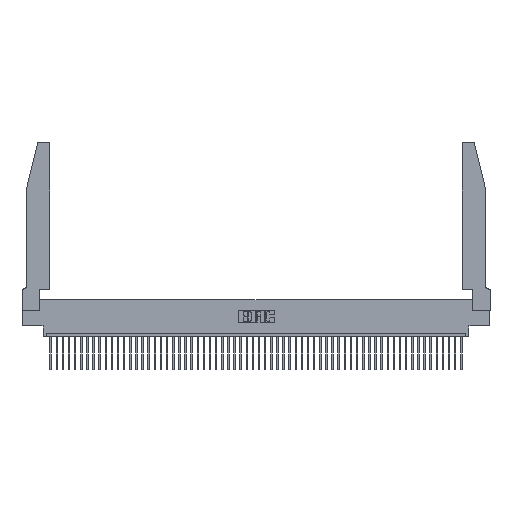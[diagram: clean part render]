
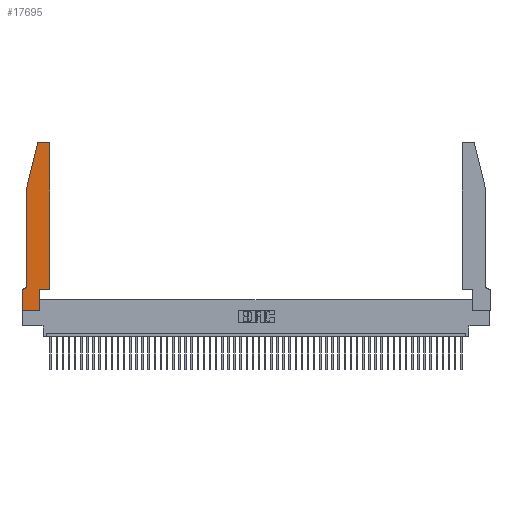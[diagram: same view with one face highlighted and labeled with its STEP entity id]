
A CAD part, top view. The second image highlights one B-rep face of the part: STEP entity #17695.
In plain terms, the highlighted planar face has unit normal (0, 0, 1).
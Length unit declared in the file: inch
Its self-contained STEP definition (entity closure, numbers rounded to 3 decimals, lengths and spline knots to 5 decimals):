
#689 = ORIENTED_EDGE ( 'NONE', *, *, #12841, .T. ) ;
#898 = DIRECTION ( 'NONE',  ( 0., 0., 1. ) ) ;
#978 = CARTESIAN_POINT ( 'NONE',  ( 0., 0., 0.37 ) ) ;
#1349 = CARTESIAN_POINT ( 'NONE',  ( 0.0755, 2., 0.37 ) ) ;
#2173 = CARTESIAN_POINT ( 'NONE',  ( 0.0755, 0.42, 0.37 ) ) ;
#2693 = DIRECTION ( 'NONE',  ( 0., 0., 1. ) ) ;
#2873 = VECTOR ( 'NONE', #14206, 39.37008 ) ;
#4176 = CIRCLE ( 'NONE', #28029, 0.03 ) ;
#4254 = CARTESIAN_POINT ( 'NONE',  ( 0., 0., 0.37 ) ) ;
#4898 = LINE ( 'NONE', #13164, #34151 ) ;
#6686 = VERTEX_POINT ( 'NONE', #15006 ) ;
#6772 = DIRECTION ( 'NONE',  ( 1., 0., 0. ) ) ;
#8226 = ORIENTED_EDGE ( 'NONE', *, *, #20039, .T. ) ;
#8615 = ORIENTED_EDGE ( 'NONE', *, *, #48968, .T. ) ;
#8838 = CARTESIAN_POINT ( 'NONE',  ( 0.2865, 0.35, 0.37 ) ) ;
#10948 = ORIENTED_EDGE ( 'NONE', *, *, #19358, .T. ) ;
#11020 = DIRECTION ( 'NONE',  ( 1., 0., 0. ) ) ;
#11480 = VECTOR ( 'NONE', #26104, 39.37008 ) ;
#11976 = EDGE_CURVE ( 'NONE', #18984, #33831, #35583, .T. ) ;
#12631 = FACE_OUTER_BOUND ( 'NONE', #30611, .T. ) ;
#12687 = CARTESIAN_POINT ( 'NONE',  ( 0.2605, 2.75, 0.37 ) ) ;
#12841 = EDGE_CURVE ( 'NONE', #29000, #18984, #4898, .T. ) ;
#13164 = CARTESIAN_POINT ( 'NONE',  ( 0.2865, 0.35, 0.37 ) ) ;
#13382 = VECTOR ( 'NONE', #45969, 39.37008 ) ;
#13775 = ORIENTED_EDGE ( 'NONE', *, *, #36613, .T. ) ;
#14206 = DIRECTION ( 'NONE',  ( 1., 0., 0. ) ) ;
#14802 = DIRECTION ( 'NONE',  ( 1., 0., 0. ) ) ;
#15006 = CARTESIAN_POINT ( 'NONE',  ( 0.0055, 0.35, 0.37 ) ) ;
#15253 = CARTESIAN_POINT ( 'NONE',  ( 0.4205, 2.72, 0.37 ) ) ;
#15315 = CARTESIAN_POINT ( 'NONE',  ( 0., 0.35, 0.37 ) ) ;
#16146 = DIRECTION ( 'NONE',  ( 0., 0., -1. ) ) ;
#16228 = VERTEX_POINT ( 'NONE', #49581 ) ;
#16940 = AXIS2_PLACEMENT_3D ( 'NONE', #43182, #2693, #6772 ) ;
#17523 = LINE ( 'NONE', #24568, #25081 ) ;
#17695 = ADVANCED_FACE ( 'NONE', ( #12631 ), #18202, .T. ) ;
#17924 = CARTESIAN_POINT ( 'NONE',  ( 0.0755, 2., 0.37 ) ) ;
#18202 = PLANE ( 'NONE',  #19454 ) ;
#18301 = EDGE_CURVE ( 'NONE', #24380, #6686, #25155, .T. ) ;
#18719 = VECTOR ( 'NONE', #29049, 39.37008 ) ;
#18984 = VERTEX_POINT ( 'NONE', #8838 ) ;
#19358 = EDGE_CURVE ( 'NONE', #36902, #28994, #4176, .T. ) ;
#19454 = AXIS2_PLACEMENT_3D ( 'NONE', #52340, #898, #14802 ) ;
#19615 = ORIENTED_EDGE ( 'NONE', *, *, #11976, .T. ) ;
#20039 = EDGE_CURVE ( 'NONE', #51931, #29000, #47998, .T. ) ;
#20915 = EDGE_CURVE ( 'NONE', #23450, #16228, #42098, .T. ) ;
#22613 = CARTESIAN_POINT ( 'NONE',  ( 0.284, 2.75, 0.37 ) ) ;
#23111 = DIRECTION ( 'NONE',  ( 0., 0., 1. ) ) ;
#23450 = VERTEX_POINT ( 'NONE', #22613 ) ;
#24380 = VERTEX_POINT ( 'NONE', #2173 ) ;
#24568 = CARTESIAN_POINT ( 'NONE',  ( 0.0755, 0.35, 0.37 ) ) ;
#25081 = VECTOR ( 'NONE', #33972, 39.37008 ) ;
#25155 = CIRCLE ( 'NONE', #28321, 0.07 ) ;
#25313 = ORIENTED_EDGE ( 'NONE', *, *, #18301, .T. ) ;
#25904 = CARTESIAN_POINT ( 'NONE',  ( 0., 0., 0.37 ) ) ;
#25976 = DIRECTION ( 'NONE',  ( 0., 1., 0. ) ) ;
#26104 = DIRECTION ( 'NONE',  ( 0., 1., 0. ) ) ;
#26651 = LINE ( 'NONE', #17924, #49461 ) ;
#27323 = CARTESIAN_POINT ( 'NONE',  ( 0.4505, 0.35, 0.37 ) ) ;
#28029 = AXIS2_PLACEMENT_3D ( 'NONE', #15253, #23111, #11020 ) ;
#28321 = AXIS2_PLACEMENT_3D ( 'NONE', #42640, #16146, #32679 ) ;
#28559 = ORIENTED_EDGE ( 'NONE', *, *, #45787, .T. ) ;
#28994 = VERTEX_POINT ( 'NONE', #38900 ) ;
#29000 = VERTEX_POINT ( 'NONE', #51292 ) ;
#29049 = DIRECTION ( 'NONE',  ( -1., 0., 0. ) ) ;
#29093 = LINE ( 'NONE', #978, #31085 ) ;
#30507 = DIRECTION ( 'NONE',  ( 0., -1., 0. ) ) ;
#30611 = EDGE_LOOP ( 'NONE', ( #28559, #51574, #41294, #13775, #25313, #48264, #52127, #8226, #689, #19615, #8615, #10948 ) ) ;
#31085 = VECTOR ( 'NONE', #30507, 39.37008 ) ;
#32187 = EDGE_CURVE ( 'NONE', #45238, #51931, #29093, .T. ) ;
#32679 = DIRECTION ( 'NONE',  ( -1., 0., 0. ) ) ;
#33831 = VERTEX_POINT ( 'NONE', #50479 ) ;
#33949 = EDGE_CURVE ( 'NONE', #6686, #45238, #17523, .T. ) ;
#33972 = DIRECTION ( 'NONE',  ( -1., 0., 0. ) ) ;
#34151 = VECTOR ( 'NONE', #25976, 39.37008 ) ;
#35583 = LINE ( 'NONE', #27323, #41892 ) ;
#36613 = EDGE_CURVE ( 'NONE', #42756, #24380, #47185, .T. ) ;
#36902 = VERTEX_POINT ( 'NONE', #46282 ) ;
#38220 = CARTESIAN_POINT ( 'NONE',  ( 0.4505, 0.35, 0.37 ) ) ;
#38408 = DIRECTION ( 'NONE',  ( -0.239, -0.971, 0. ) ) ;
#38900 = CARTESIAN_POINT ( 'NONE',  ( 0.4205, 2.75, 0.37 ) ) ;
#41294 = ORIENTED_EDGE ( 'NONE', *, *, #48977, .T. ) ;
#41892 = VECTOR ( 'NONE', #43498, 39.37008 ) ;
#42098 = CIRCLE ( 'NONE', #16940, 0.03 ) ;
#42640 = CARTESIAN_POINT ( 'NONE',  ( 0.0055, 0.42, 0.37 ) ) ;
#42756 = VERTEX_POINT ( 'NONE', #43298 ) ;
#43182 = CARTESIAN_POINT ( 'NONE',  ( 0.284, 2.72, 0.37 ) ) ;
#43298 = CARTESIAN_POINT ( 'NONE',  ( 0.0755, 2., 0.37 ) ) ;
#43498 = DIRECTION ( 'NONE',  ( 1., 0., 0. ) ) ;
#45238 = VERTEX_POINT ( 'NONE', #15315 ) ;
#45787 = EDGE_CURVE ( 'NONE', #28994, #23450, #47373, .T. ) ;
#45969 = DIRECTION ( 'NONE',  ( 0., -1., 0. ) ) ;
#46282 = CARTESIAN_POINT ( 'NONE',  ( 0.4505, 2.72, 0.37 ) ) ;
#47185 = LINE ( 'NONE', #1349, #13382 ) ;
#47373 = LINE ( 'NONE', #12687, #18719 ) ;
#47998 = LINE ( 'NONE', #25904, #2873 ) ;
#48264 = ORIENTED_EDGE ( 'NONE', *, *, #33949, .T. ) ;
#48968 = EDGE_CURVE ( 'NONE', #33831, #36902, #49509, .T. ) ;
#48977 = EDGE_CURVE ( 'NONE', #16228, #42756, #26651, .T. ) ;
#49461 = VECTOR ( 'NONE', #38408, 39.37008 ) ;
#49509 = LINE ( 'NONE', #38220, #11480 ) ;
#49581 = CARTESIAN_POINT ( 'NONE',  ( 0.25487, 2.72718, 0.37 ) ) ;
#50479 = CARTESIAN_POINT ( 'NONE',  ( 0.4505, 0.35, 0.37 ) ) ;
#51292 = CARTESIAN_POINT ( 'NONE',  ( 0.2865, 0., 0.37 ) ) ;
#51574 = ORIENTED_EDGE ( 'NONE', *, *, #20915, .T. ) ;
#51931 = VERTEX_POINT ( 'NONE', #4254 ) ;
#52127 = ORIENTED_EDGE ( 'NONE', *, *, #32187, .T. ) ;
#52340 = CARTESIAN_POINT ( 'NONE',  ( 0., 0.35, 0.37 ) ) ;
